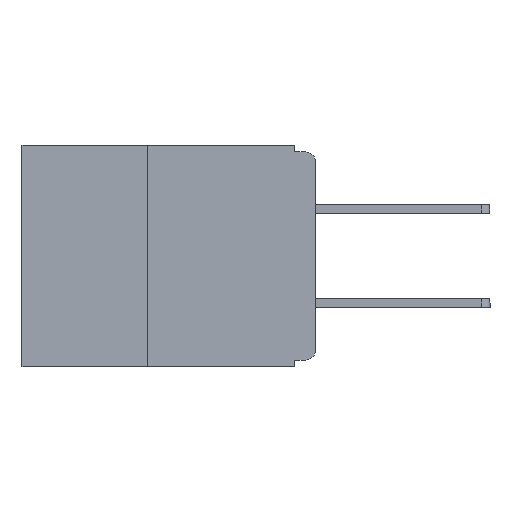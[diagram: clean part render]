
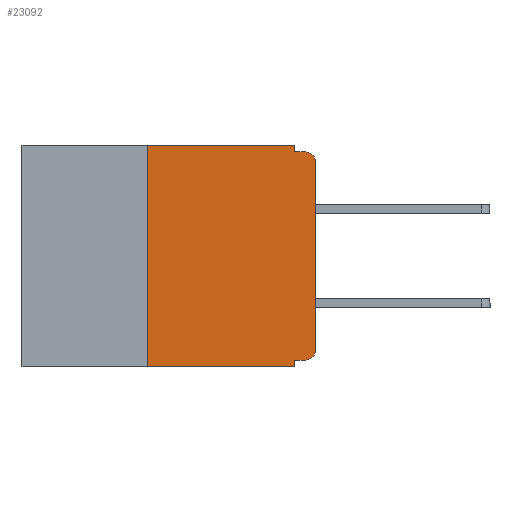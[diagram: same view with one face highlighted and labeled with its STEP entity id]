
A CAD part, left-side view. The second image highlights one B-rep face of the part: STEP entity #23092.
In plain terms, the highlighted planar face has unit normal (-1, 0, 0).
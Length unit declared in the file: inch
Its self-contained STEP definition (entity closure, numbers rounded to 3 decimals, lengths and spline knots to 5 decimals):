
#156 = DIRECTION ( 'NONE',  ( -1., 0., 0. ) ) ;
#750 = VERTEX_POINT ( 'NONE', #19431 ) ;
#1882 = EDGE_CURVE ( 'NONE', #25020, #1889, #16050, .T. ) ;
#1889 = VERTEX_POINT ( 'NONE', #11507 ) ;
#3205 = VECTOR ( 'NONE', #3302, 39.37008 ) ;
#3302 = DIRECTION ( 'NONE',  ( 0., 0., -1. ) ) ;
#4117 = EDGE_CURVE ( 'NONE', #15410, #15295, #4137, .T. ) ;
#4126 = AXIS2_PLACEMENT_3D ( 'NONE', #14912, #156, #17348 ) ;
#4137 = LINE ( 'NONE', #29502, #16378 ) ;
#4679 = EDGE_CURVE ( 'NONE', #750, #25691, #7615, .T. ) ;
#5042 = PLANE ( 'NONE',  #12320 ) ;
#5358 = CARTESIAN_POINT ( 'NONE',  ( 0., 0.031, 0. ) ) ;
#6075 = CARTESIAN_POINT ( 'NONE',  ( 0., 0.031, -0.33 ) ) ;
#6319 = LINE ( 'NONE', #16758, #30556 ) ;
#6526 = DIRECTION ( 'NONE',  ( 0., 1., 0. ) ) ;
#6834 = ORIENTED_EDGE ( 'NONE', *, *, #11330, .F. ) ;
#7046 = CIRCLE ( 'NONE', #12660, 0.015 ) ;
#7565 = DIRECTION ( 'NONE',  ( 1., 0., 0. ) ) ;
#7615 = LINE ( 'NONE', #22186, #20389 ) ;
#7819 = EDGE_LOOP ( 'NONE', ( #17531, #28124, #9346, #10165, #6834, #20628, #23822, #27083, #15736, #29404 ) ) ;
#8424 = CARTESIAN_POINT ( 'NONE',  ( 0., 0.015, -0.32 ) ) ;
#8528 = CARTESIAN_POINT ( 'NONE',  ( 0., 0.015, -0.305 ) ) ;
#8959 = CARTESIAN_POINT ( 'NONE',  ( 0., 0., -0.32 ) ) ;
#9346 = ORIENTED_EDGE ( 'NONE', *, *, #18142, .F. ) ;
#10165 = ORIENTED_EDGE ( 'NONE', *, *, #4117, .F. ) ;
#10593 = LINE ( 'NONE', #20382, #3205 ) ;
#10819 = VECTOR ( 'NONE', #22963, 39.37008 ) ;
#10954 = DIRECTION ( 'NONE',  ( 0., 0., -1. ) ) ;
#11330 = EDGE_CURVE ( 'NONE', #1889, #15410, #11562, .T. ) ;
#11470 = CARTESIAN_POINT ( 'NONE',  ( 0., 0.437, 0. ) ) ;
#11507 = CARTESIAN_POINT ( 'NONE',  ( 0., 0.25, 0. ) ) ;
#11562 = LINE ( 'NONE', #11470, #29362 ) ;
#12320 = AXIS2_PLACEMENT_3D ( 'NONE', #21908, #7565, #24247 ) ;
#12660 = AXIS2_PLACEMENT_3D ( 'NONE', #8528, #25115, #10954 ) ;
#14085 = CIRCLE ( 'NONE', #4126, 0.015 ) ;
#14143 = LINE ( 'NONE', #8959, #18283 ) ;
#14264 = CARTESIAN_POINT ( 'NONE',  ( 0., 0.25, -0.33 ) ) ;
#14434 = CARTESIAN_POINT ( 'NONE',  ( 0., 0., -0.025 ) ) ;
#14675 = CARTESIAN_POINT ( 'NONE',  ( 0., 0.031, -0.01 ) ) ;
#14912 = CARTESIAN_POINT ( 'NONE',  ( 0., 0.015, -0.025 ) ) ;
#15295 = VERTEX_POINT ( 'NONE', #14675 ) ;
#15410 = VERTEX_POINT ( 'NONE', #5358 ) ;
#15736 = ORIENTED_EDGE ( 'NONE', *, *, #22208, .F. ) ;
#15873 = CARTESIAN_POINT ( 'NONE',  ( 0., 0., -0.01 ) ) ;
#16050 = LINE ( 'NONE', #21176, #27680 ) ;
#16259 = EDGE_CURVE ( 'NONE', #19846, #750, #7046, .T. ) ;
#16378 = VECTOR ( 'NONE', #20136, 39.37008 ) ;
#16758 = CARTESIAN_POINT ( 'NONE',  ( 0., 0.437, -0.33 ) ) ;
#17217 = LINE ( 'NONE', #15873, #10819 ) ;
#17348 = DIRECTION ( 'NONE',  ( 0., 0., -1. ) ) ;
#17531 = ORIENTED_EDGE ( 'NONE', *, *, #4679, .T. ) ;
#18097 = VERTEX_POINT ( 'NONE', #6075 ) ;
#18142 = EDGE_CURVE ( 'NONE', #15295, #30541, #17217, .T. ) ;
#18283 = VECTOR ( 'NONE', #6526, 39.37008 ) ;
#19248 = DIRECTION ( 'NONE',  ( 0., -1., 0. ) ) ;
#19431 = CARTESIAN_POINT ( 'NONE',  ( 0., 0., -0.305 ) ) ;
#19846 = VERTEX_POINT ( 'NONE', #8424 ) ;
#20136 = DIRECTION ( 'NONE',  ( 0., 0., -1. ) ) ;
#20382 = CARTESIAN_POINT ( 'NONE',  ( 0., 0.031, -0.33 ) ) ;
#20389 = VECTOR ( 'NONE', #22144, 39.37008 ) ;
#20628 = ORIENTED_EDGE ( 'NONE', *, *, #1882, .F. ) ;
#20976 = CARTESIAN_POINT ( 'NONE',  ( 0., 0.031, -0.32 ) ) ;
#21079 = DIRECTION ( 'NONE',  ( 0., 0., 1. ) ) ;
#21176 = CARTESIAN_POINT ( 'NONE',  ( 0., 0.25, -0.33 ) ) ;
#21908 = CARTESIAN_POINT ( 'NONE',  ( 0., 0.437, 0. ) ) ;
#22144 = DIRECTION ( 'NONE',  ( 0., 0., 1. ) ) ;
#22186 = CARTESIAN_POINT ( 'NONE',  ( 0., 0., 0. ) ) ;
#22208 = EDGE_CURVE ( 'NONE', #19846, #29936, #14143, .T. ) ;
#22963 = DIRECTION ( 'NONE',  ( 0., -1., 0. ) ) ;
#23092 = ADVANCED_FACE ( 'NONE', ( #25847 ), #5042, .F. ) ;
#23822 = ORIENTED_EDGE ( 'NONE', *, *, #25694, .T. ) ;
#24247 = DIRECTION ( 'NONE',  ( 0., 0., -1. ) ) ;
#25020 = VERTEX_POINT ( 'NONE', #14264 ) ;
#25115 = DIRECTION ( 'NONE',  ( -1., 0., 0. ) ) ;
#25580 = DIRECTION ( 'NONE',  ( 0., -1., 0. ) ) ;
#25691 = VERTEX_POINT ( 'NONE', #14434 ) ;
#25694 = EDGE_CURVE ( 'NONE', #25020, #18097, #6319, .T. ) ;
#25847 = FACE_OUTER_BOUND ( 'NONE', #7819, .T. ) ;
#27083 = ORIENTED_EDGE ( 'NONE', *, *, #29791, .F. ) ;
#27621 = EDGE_CURVE ( 'NONE', #25691, #30541, #14085, .T. ) ;
#27680 = VECTOR ( 'NONE', #21079, 39.37008 ) ;
#28053 = CARTESIAN_POINT ( 'NONE',  ( 0., 0.015, -0.01 ) ) ;
#28124 = ORIENTED_EDGE ( 'NONE', *, *, #27621, .T. ) ;
#29362 = VECTOR ( 'NONE', #25580, 39.37008 ) ;
#29404 = ORIENTED_EDGE ( 'NONE', *, *, #16259, .T. ) ;
#29502 = CARTESIAN_POINT ( 'NONE',  ( 0., 0.031, 0. ) ) ;
#29791 = EDGE_CURVE ( 'NONE', #29936, #18097, #10593, .T. ) ;
#29936 = VERTEX_POINT ( 'NONE', #20976 ) ;
#30541 = VERTEX_POINT ( 'NONE', #28053 ) ;
#30556 = VECTOR ( 'NONE', #19248, 39.37008 ) ;
